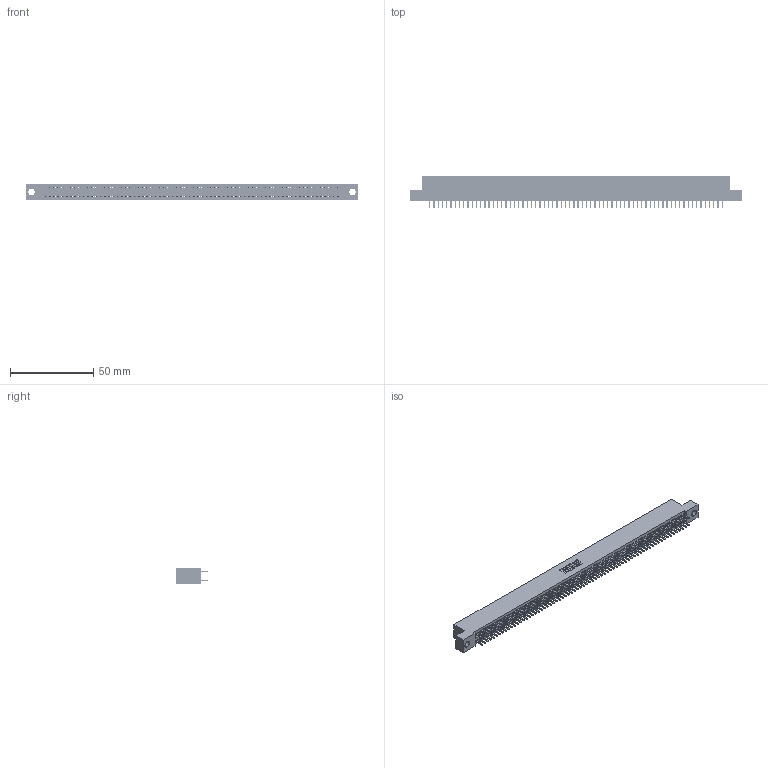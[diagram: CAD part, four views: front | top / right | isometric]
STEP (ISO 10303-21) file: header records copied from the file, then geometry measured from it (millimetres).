
FILE_DESCRIPTION (( 'STEP AP203' ), '1' );
FILE_NAME ('345-140-520-204.STEP', '2021-05-26T00:40:18', ( '' ), ( '' ), 'SwSTEP 2.0', 'SolidWorks 2020', '' );
FILE_SCHEMA (( 'CONFIG_CONTROL_DESIGN' ));
Length unit declared in the file: inch
Products named in the file (3): 345-140-520-204; 345 Part_Flush Mounting Lugs - 0.156 Dia-TI; 345-292-001_345-293-120
Assembly tree (141 placements, depth 2):
  345-140-520-204
    345 Part_Flush Mounting Lugs - 0.156 Dia-TI
    345-292-001_345-293-120  x140
Bounding box: 199.01 x 19.68 x 9.4 mm (x, y, z)
Volume: 19424.3 mm3; surface area: 28975.4 mm2
Topology: 141 solids, 141 shells, 7700 faces, 22357 edges, 14530 vertices
Faces by surface type: plane 4994, cylinder 2706
Entity records: 51687 total; most frequent: CARTESIAN_POINT 8654, ORIENTED_EDGE 8574, DIRECTION 7583, EDGE_CURVE 4287, VECTOR 3871, LINE 3871, VERTEX_POINT 2854, AXIS2_PLACEMENT_3D 1856
